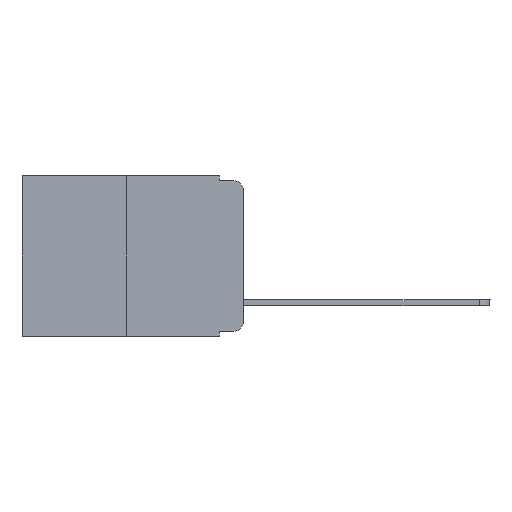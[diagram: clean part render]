
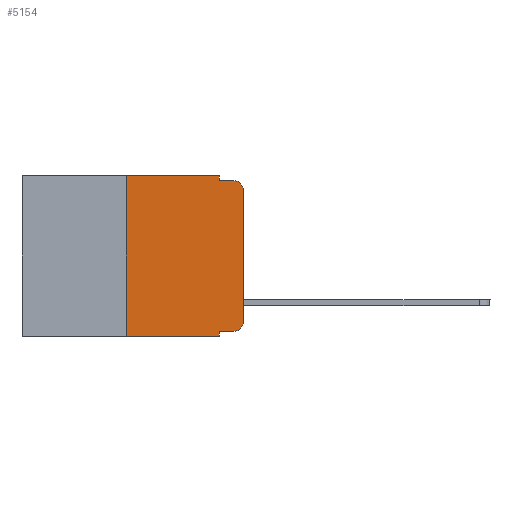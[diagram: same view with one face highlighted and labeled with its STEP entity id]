
A CAD part, left-side view. The second image highlights one B-rep face of the part: STEP entity #5154.
In plain terms, the highlighted planar face has unit normal (-1, 0, 0).
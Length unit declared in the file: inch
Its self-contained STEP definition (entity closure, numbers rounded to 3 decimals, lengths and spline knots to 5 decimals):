
#124 = EDGE_CURVE ( 'NONE', #6475, #1956, #4953, .T. ) ;
#466 = EDGE_CURVE ( 'NONE', #642, #6475, #15088, .T. ) ;
#642 = VERTEX_POINT ( 'NONE', #9997 ) ;
#1657 = VERTEX_POINT ( 'NONE', #19979 ) ;
#1679 = AXIS2_PLACEMENT_3D ( 'NONE', #8108, #19432, #4722 ) ;
#1745 = CARTESIAN_POINT ( 'NONE',  ( 0., 0.051, -0.01 ) ) ;
#1956 = VERTEX_POINT ( 'NONE', #1745 ) ;
#2562 = VECTOR ( 'NONE', #19609, 39.37008 ) ;
#3520 = CARTESIAN_POINT ( 'NONE',  ( 0., 0.02, -0.333 ) ) ;
#4093 = CARTESIAN_POINT ( 'NONE',  ( 0., 0.051, -0.333 ) ) ;
#4585 = AXIS2_PLACEMENT_3D ( 'NONE', #13688, #8868, #20419 ) ;
#4722 = DIRECTION ( 'NONE',  ( 0., 0., -1. ) ) ;
#4928 = VERTEX_POINT ( 'NONE', #9116 ) ;
#4953 = LINE ( 'NONE', #16993, #10507 ) ;
#5154 = ADVANCED_FACE ( 'NONE', ( #8750 ), #14567, .F. ) ;
#5478 = CARTESIAN_POINT ( 'NONE',  ( 0., 0., -0.03 ) ) ;
#5531 = CARTESIAN_POINT ( 'NONE',  ( 0., 0.25, 0. ) ) ;
#5668 = VECTOR ( 'NONE', #15188, 39.37008 ) ;
#5731 = CIRCLE ( 'NONE', #4585, 0.02 ) ;
#6008 = DIRECTION ( 'NONE',  ( -1., 0., 0. ) ) ;
#6475 = VERTEX_POINT ( 'NONE', #13882 ) ;
#6819 = EDGE_CURVE ( 'NONE', #17001, #11558, #11939, .T. ) ;
#6823 = ORIENTED_EDGE ( 'NONE', *, *, #124, .F. ) ;
#7571 = EDGE_CURVE ( 'NONE', #11558, #4928, #5731, .T. ) ;
#7618 = DIRECTION ( 'NONE',  ( 0., -1., 0. ) ) ;
#8108 = CARTESIAN_POINT ( 'NONE',  ( 0., 0.473, 0. ) ) ;
#8465 = LINE ( 'NONE', #16420, #15581 ) ;
#8561 = CARTESIAN_POINT ( 'NONE',  ( 0., 0.051, -0.333 ) ) ;
#8654 = LINE ( 'NONE', #19884, #2562 ) ;
#8750 = FACE_OUTER_BOUND ( 'NONE', #14574, .T. ) ;
#8868 = DIRECTION ( 'NONE',  ( -1., 0., 0. ) ) ;
#8876 = LINE ( 'NONE', #4093, #9147 ) ;
#9059 = DIRECTION ( 'NONE',  ( 0., 0., -1. ) ) ;
#9116 = CARTESIAN_POINT ( 'NONE',  ( 0., 0.02, -0.01 ) ) ;
#9147 = VECTOR ( 'NONE', #18687, 39.37008 ) ;
#9655 = EDGE_CURVE ( 'NONE', #11844, #17001, #12551, .T. ) ;
#9708 = LINE ( 'NONE', #5531, #5668 ) ;
#9735 = DIRECTION ( 'NONE',  ( 0., 0., 1. ) ) ;
#9942 = DIRECTION ( 'NONE',  ( 0., -1., 0. ) ) ;
#9997 = CARTESIAN_POINT ( 'NONE',  ( 0., 0.25, 0. ) ) ;
#10052 = VERTEX_POINT ( 'NONE', #12067 ) ;
#10507 = VECTOR ( 'NONE', #9059, 39.37008 ) ;
#10756 = VECTOR ( 'NONE', #9942, 39.37008 ) ;
#11390 = DIRECTION ( 'NONE',  ( 0., -1., 0. ) ) ;
#11558 = VERTEX_POINT ( 'NONE', #5478 ) ;
#11751 = ORIENTED_EDGE ( 'NONE', *, *, #7571, .T. ) ;
#11844 = VERTEX_POINT ( 'NONE', #3520 ) ;
#11939 = LINE ( 'NONE', #16396, #19808 ) ;
#11977 = LINE ( 'NONE', #12512, #13267 ) ;
#12067 = CARTESIAN_POINT ( 'NONE',  ( 0., 0.25, -0.343 ) ) ;
#12315 = EDGE_CURVE ( 'NONE', #18907, #1657, #8654, .T. ) ;
#12512 = CARTESIAN_POINT ( 'NONE',  ( 0., 0.473, -0.343 ) ) ;
#12551 = CIRCLE ( 'NONE', #14131, 0.02 ) ;
#12621 = CARTESIAN_POINT ( 'NONE',  ( 0., 0.02, -0.313 ) ) ;
#13079 = EDGE_CURVE ( 'NONE', #18907, #11844, #8876, .T. ) ;
#13267 = VECTOR ( 'NONE', #7618, 39.37008 ) ;
#13688 = CARTESIAN_POINT ( 'NONE',  ( 0., 0.02, -0.03 ) ) ;
#13882 = CARTESIAN_POINT ( 'NONE',  ( 0., 0.051, 0. ) ) ;
#14131 = AXIS2_PLACEMENT_3D ( 'NONE', #12621, #6008, #20462 ) ;
#14567 = PLANE ( 'NONE',  #1679 ) ;
#14574 = EDGE_LOOP ( 'NONE', ( #19162, #11751, #19714, #6823, #19461, #18862, #15266, #18235, #16733, #15414 ) ) ;
#14665 = CARTESIAN_POINT ( 'NONE',  ( 0., 0.473, 0. ) ) ;
#15088 = LINE ( 'NONE', #14665, #10756 ) ;
#15188 = DIRECTION ( 'NONE',  ( 0., 0., 1. ) ) ;
#15266 = ORIENTED_EDGE ( 'NONE', *, *, #17954, .T. ) ;
#15414 = ORIENTED_EDGE ( 'NONE', *, *, #9655, .T. ) ;
#15581 = VECTOR ( 'NONE', #11390, 39.37008 ) ;
#16396 = CARTESIAN_POINT ( 'NONE',  ( 0., 0., 0. ) ) ;
#16420 = CARTESIAN_POINT ( 'NONE',  ( 0., 0.051, -0.01 ) ) ;
#16733 = ORIENTED_EDGE ( 'NONE', *, *, #13079, .T. ) ;
#16993 = CARTESIAN_POINT ( 'NONE',  ( 0., 0.051, 0. ) ) ;
#17001 = VERTEX_POINT ( 'NONE', #17009 ) ;
#17009 = CARTESIAN_POINT ( 'NONE',  ( 0., 0., -0.313 ) ) ;
#17954 = EDGE_CURVE ( 'NONE', #10052, #1657, #11977, .T. ) ;
#18235 = ORIENTED_EDGE ( 'NONE', *, *, #12315, .F. ) ;
#18402 = EDGE_CURVE ( 'NONE', #10052, #642, #9708, .T. ) ;
#18422 = EDGE_CURVE ( 'NONE', #1956, #4928, #8465, .T. ) ;
#18687 = DIRECTION ( 'NONE',  ( 0., -1., 0. ) ) ;
#18862 = ORIENTED_EDGE ( 'NONE', *, *, #18402, .F. ) ;
#18907 = VERTEX_POINT ( 'NONE', #8561 ) ;
#19162 = ORIENTED_EDGE ( 'NONE', *, *, #6819, .T. ) ;
#19432 = DIRECTION ( 'NONE',  ( 1., 0., 0. ) ) ;
#19461 = ORIENTED_EDGE ( 'NONE', *, *, #466, .F. ) ;
#19609 = DIRECTION ( 'NONE',  ( 0., 0., -1. ) ) ;
#19714 = ORIENTED_EDGE ( 'NONE', *, *, #18422, .F. ) ;
#19808 = VECTOR ( 'NONE', #9735, 39.37008 ) ;
#19884 = CARTESIAN_POINT ( 'NONE',  ( 0., 0.051, 0. ) ) ;
#19979 = CARTESIAN_POINT ( 'NONE',  ( 0., 0.051, -0.343 ) ) ;
#20419 = DIRECTION ( 'NONE',  ( 0., 0., -1. ) ) ;
#20462 = DIRECTION ( 'NONE',  ( 0., 0., -1. ) ) ;
